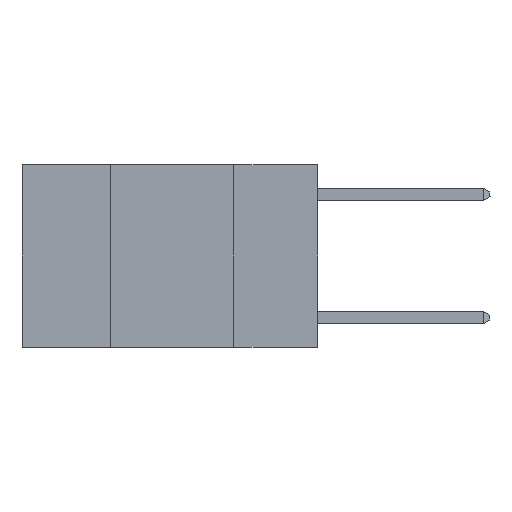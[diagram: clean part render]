
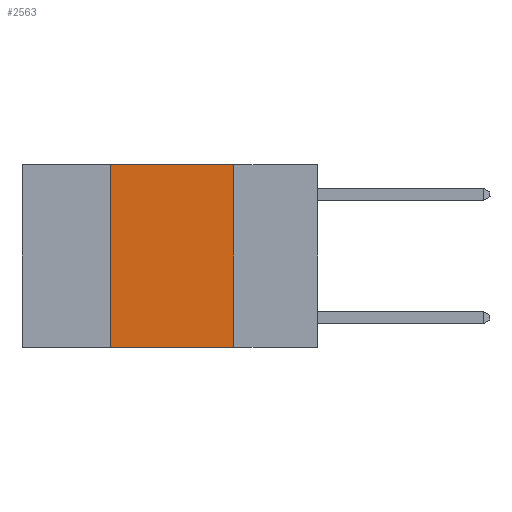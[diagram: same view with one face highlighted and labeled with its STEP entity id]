
A CAD part, left-side view. The second image highlights one B-rep face of the part: STEP entity #2563.
In plain terms, the highlighted planar face has unit normal (-1, 0, 0).
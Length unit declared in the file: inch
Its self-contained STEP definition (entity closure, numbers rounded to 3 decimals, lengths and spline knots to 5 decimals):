
#78 = CARTESIAN_POINT ( 'NONE',  ( 0., 0.6, 0. ) ) ;
#854 = EDGE_CURVE ( 'NONE', #5870, #2933, #4439, .T. ) ;
#1208 = DIRECTION ( 'NONE',  ( 0., 0., 1. ) ) ;
#1323 = CARTESIAN_POINT ( 'NONE',  ( 0., 0.42, 0. ) ) ;
#1417 = EDGE_CURVE ( 'NONE', #8503, #4753, #9872, .T. ) ;
#1499 = CARTESIAN_POINT ( 'NONE',  ( 0., 0.17, -0.37 ) ) ;
#1672 = CARTESIAN_POINT ( 'NONE',  ( 0., 0.17, 0. ) ) ;
#2047 = DIRECTION ( 'NONE',  ( 1., 0., 0. ) ) ;
#2108 = AXIS2_PLACEMENT_3D ( 'NONE', #8194, #2047, #6685 ) ;
#2297 = DIRECTION ( 'NONE',  ( 0., 0., -1. ) ) ;
#2448 = DIRECTION ( 'NONE',  ( 0., -1., 0. ) ) ;
#2563 = ADVANCED_FACE ( 'NONE', ( #9823 ), #3640, .F. ) ;
#2855 = CARTESIAN_POINT ( 'NONE',  ( 0., 0.42, -0.37 ) ) ;
#2930 = EDGE_CURVE ( 'NONE', #5870, #4753, #6463, .T. ) ;
#2933 = VERTEX_POINT ( 'NONE', #4123 ) ;
#3640 = PLANE ( 'NONE',  #2108 ) ;
#3657 = VECTOR ( 'NONE', #1208, 39.37008 ) ;
#3710 = VECTOR ( 'NONE', #5680, 39.37008 ) ;
#3939 = LINE ( 'NONE', #78, #6149 ) ;
#4123 = CARTESIAN_POINT ( 'NONE',  ( 0., 0.42, 0. ) ) ;
#4439 = LINE ( 'NONE', #1323, #3657 ) ;
#4753 = VERTEX_POINT ( 'NONE', #1499 ) ;
#5427 = CARTESIAN_POINT ( 'NONE',  ( 0., 0.17, 0. ) ) ;
#5680 = DIRECTION ( 'NONE',  ( 0., -1., 0. ) ) ;
#5870 = VERTEX_POINT ( 'NONE', #2855 ) ;
#6149 = VECTOR ( 'NONE', #2448, 39.37008 ) ;
#6463 = LINE ( 'NONE', #9490, #3710 ) ;
#6501 = ORIENTED_EDGE ( 'NONE', *, *, #854, .F. ) ;
#6685 = DIRECTION ( 'NONE',  ( 0., 0., -1. ) ) ;
#7082 = EDGE_LOOP ( 'NONE', ( #7382, #9730, #6501, #8411 ) ) ;
#7382 = ORIENTED_EDGE ( 'NONE', *, *, #1417, .F. ) ;
#8194 = CARTESIAN_POINT ( 'NONE',  ( 0., 0.6, 0. ) ) ;
#8411 = ORIENTED_EDGE ( 'NONE', *, *, #2930, .T. ) ;
#8475 = EDGE_CURVE ( 'NONE', #2933, #8503, #3939, .T. ) ;
#8503 = VERTEX_POINT ( 'NONE', #1672 ) ;
#8602 = VECTOR ( 'NONE', #2297, 39.37008 ) ;
#9490 = CARTESIAN_POINT ( 'NONE',  ( 0., 0.6, -0.37 ) ) ;
#9730 = ORIENTED_EDGE ( 'NONE', *, *, #8475, .F. ) ;
#9823 = FACE_OUTER_BOUND ( 'NONE', #7082, .T. ) ;
#9872 = LINE ( 'NONE', #5427, #8602 ) ;
